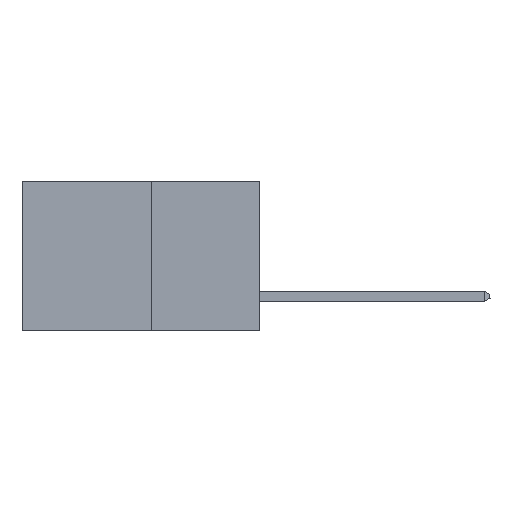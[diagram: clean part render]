
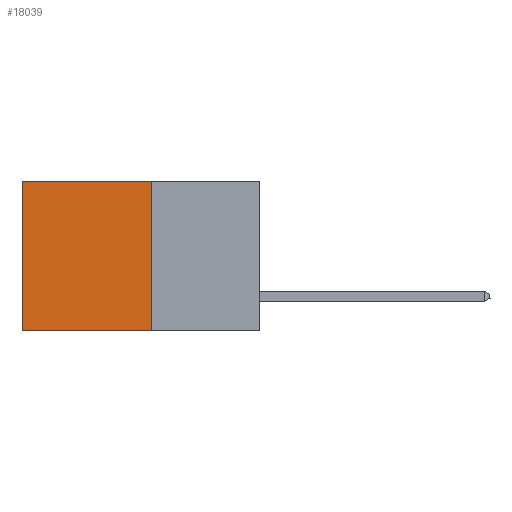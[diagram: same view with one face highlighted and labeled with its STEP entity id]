
A CAD part, left-side view. The second image highlights one B-rep face of the part: STEP entity #18039.
In plain terms, the highlighted planar face has unit normal (-1, 0, 0).
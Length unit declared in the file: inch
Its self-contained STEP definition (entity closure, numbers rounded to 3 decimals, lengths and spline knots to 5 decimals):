
#288 = LINE ( 'NONE', #13464, #17113 ) ;
#491 = EDGE_CURVE ( 'NONE', #16204, #4393, #5868, .T. ) ;
#1223 = VECTOR ( 'NONE', #8731, 39.37008 ) ;
#1231 = CARTESIAN_POINT ( 'NONE',  ( 0.277, 0.59, 0. ) ) ;
#2095 = ORIENTED_EDGE ( 'NONE', *, *, #491, .T. ) ;
#2203 = CARTESIAN_POINT ( 'NONE',  ( 0.277, 0.27, 0. ) ) ;
#2994 = DIRECTION ( 'NONE',  ( 0., 0., -1. ) ) ;
#3552 = ORIENTED_EDGE ( 'NONE', *, *, #7532, .T. ) ;
#3937 = CARTESIAN_POINT ( 'NONE',  ( 0.277, 0.27, -0.37 ) ) ;
#4393 = VERTEX_POINT ( 'NONE', #1231 ) ;
#5076 = EDGE_LOOP ( 'NONE', ( #3552, #5728, #16579, #2095 ) ) ;
#5728 = ORIENTED_EDGE ( 'NONE', *, *, #10687, .F. ) ;
#5868 = LINE ( 'NONE', #2203, #1223 ) ;
#7532 = EDGE_CURVE ( 'NONE', #4393, #16655, #7710, .T. ) ;
#7710 = LINE ( 'NONE', #16705, #11568 ) ;
#7732 = FACE_OUTER_BOUND ( 'NONE', #5076, .T. ) ;
#8625 = DIRECTION ( 'NONE',  ( 0., 0., -1. ) ) ;
#8665 = EDGE_CURVE ( 'NONE', #16204, #8839, #19566, .T. ) ;
#8731 = DIRECTION ( 'NONE',  ( 0., 1., 0. ) ) ;
#8839 = VERTEX_POINT ( 'NONE', #13793 ) ;
#10687 = EDGE_CURVE ( 'NONE', #8839, #16655, #288, .T. ) ;
#11568 = VECTOR ( 'NONE', #18355, 39.37008 ) ;
#11877 = AXIS2_PLACEMENT_3D ( 'NONE', #16868, #18537, #8625 ) ;
#12042 = CARTESIAN_POINT ( 'NONE',  ( 0.277, 0.59, -0.37 ) ) ;
#13464 = CARTESIAN_POINT ( 'NONE',  ( 0.277, 0.27, -0.37 ) ) ;
#13793 = CARTESIAN_POINT ( 'NONE',  ( 0.277, 0.27, -0.37 ) ) ;
#15105 = VECTOR ( 'NONE', #2994, 39.37008 ) ;
#15511 = CARTESIAN_POINT ( 'NONE',  ( 0.277, 0.27, 0. ) ) ;
#16204 = VERTEX_POINT ( 'NONE', #15511 ) ;
#16579 = ORIENTED_EDGE ( 'NONE', *, *, #8665, .F. ) ;
#16655 = VERTEX_POINT ( 'NONE', #12042 ) ;
#16705 = CARTESIAN_POINT ( 'NONE',  ( 0.277, 0.59, -0.37 ) ) ;
#16808 = DIRECTION ( 'NONE',  ( 0., 1., 0. ) ) ;
#16868 = CARTESIAN_POINT ( 'NONE',  ( 0.277, 0.27, -0.37 ) ) ;
#17113 = VECTOR ( 'NONE', #16808, 39.37008 ) ;
#18039 = ADVANCED_FACE ( 'NONE', ( #7732 ), #18465, .F. ) ;
#18355 = DIRECTION ( 'NONE',  ( 0., 0., -1. ) ) ;
#18465 = PLANE ( 'NONE',  #11877 ) ;
#18537 = DIRECTION ( 'NONE',  ( 1., 0., 0. ) ) ;
#19566 = LINE ( 'NONE', #3937, #15105 ) ;
